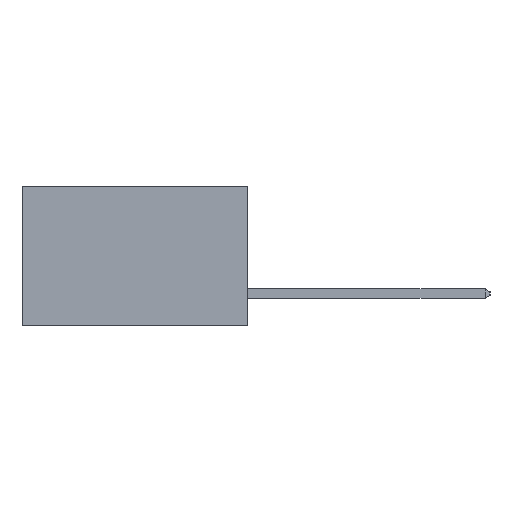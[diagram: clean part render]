
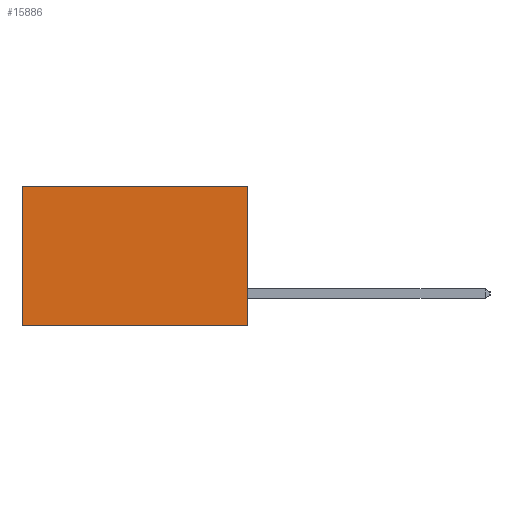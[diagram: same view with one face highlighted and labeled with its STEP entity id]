
A CAD part, left-side view. The second image highlights one B-rep face of the part: STEP entity #15886.
In plain terms, the highlighted planar face has unit normal (-1, 0, 0).
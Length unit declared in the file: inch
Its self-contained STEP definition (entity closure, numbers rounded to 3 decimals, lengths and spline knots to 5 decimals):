
#5 = DIRECTION ( 'NONE',  ( 0., 0., -1. ) ) ;
#1754 = DIRECTION ( 'NONE',  ( 0., 1., 0. ) ) ;
#2316 = VECTOR ( 'NONE', #1754, 39.37008 ) ;
#2550 = FACE_OUTER_BOUND ( 'NONE', #12616, .T. ) ;
#2822 = VERTEX_POINT ( 'NONE', #15000 ) ;
#3612 = CARTESIAN_POINT ( 'NONE',  ( 0.2615, 0., -0.37 ) ) ;
#5207 = VERTEX_POINT ( 'NONE', #10753 ) ;
#5256 = ORIENTED_EDGE ( 'NONE', *, *, #6195, .T. ) ;
#5843 = CARTESIAN_POINT ( 'NONE',  ( 0.2615, 0., -0.37 ) ) ;
#6195 = EDGE_CURVE ( 'NONE', #2822, #5207, #15801, .T. ) ;
#7599 = DIRECTION ( 'NONE',  ( 1., 0., 0. ) ) ;
#7690 = ORIENTED_EDGE ( 'NONE', *, *, #25019, .F. ) ;
#7953 = VERTEX_POINT ( 'NONE', #21336 ) ;
#8027 = CARTESIAN_POINT ( 'NONE',  ( 0.2615, 0.6, -0.37 ) ) ;
#8968 = DIRECTION ( 'NONE',  ( 0., 0., -1. ) ) ;
#10753 = CARTESIAN_POINT ( 'NONE',  ( 0.2615, 0.6, -0.37 ) ) ;
#11182 = VECTOR ( 'NONE', #5, 39.37008 ) ;
#11641 = AXIS2_PLACEMENT_3D ( 'NONE', #3612, #7599, #21332 ) ;
#11752 = EDGE_CURVE ( 'NONE', #7953, #5207, #14881, .T. ) ;
#12616 = EDGE_LOOP ( 'NONE', ( #5256, #15662, #7690, #14758 ) ) ;
#12905 = CARTESIAN_POINT ( 'NONE',  ( 0.2615, 0., -0.37 ) ) ;
#12926 = LINE ( 'NONE', #25234, #2316 ) ;
#14376 = EDGE_CURVE ( 'NONE', #24875, #2822, #12926, .T. ) ;
#14758 = ORIENTED_EDGE ( 'NONE', *, *, #14376, .T. ) ;
#14881 = LINE ( 'NONE', #5843, #19439 ) ;
#14938 = VECTOR ( 'NONE', #8968, 39.37008 ) ;
#15000 = CARTESIAN_POINT ( 'NONE',  ( 0.2615, 0.6, 0. ) ) ;
#15662 = ORIENTED_EDGE ( 'NONE', *, *, #11752, .F. ) ;
#15773 = DIRECTION ( 'NONE',  ( 0., 1., 0. ) ) ;
#15801 = LINE ( 'NONE', #8027, #11182 ) ;
#15886 = ADVANCED_FACE ( 'NONE', ( #2550 ), #19407, .F. ) ;
#19407 = PLANE ( 'NONE',  #11641 ) ;
#19439 = VECTOR ( 'NONE', #15773, 39.37008 ) ;
#20097 = LINE ( 'NONE', #12905, #14938 ) ;
#21332 = DIRECTION ( 'NONE',  ( 0., 0., -1. ) ) ;
#21336 = CARTESIAN_POINT ( 'NONE',  ( 0.2615, 0., -0.37 ) ) ;
#23979 = CARTESIAN_POINT ( 'NONE',  ( 0.2615, 0., 0. ) ) ;
#24875 = VERTEX_POINT ( 'NONE', #23979 ) ;
#25019 = EDGE_CURVE ( 'NONE', #24875, #7953, #20097, .T. ) ;
#25234 = CARTESIAN_POINT ( 'NONE',  ( 0.2615, 0., 0. ) ) ;
